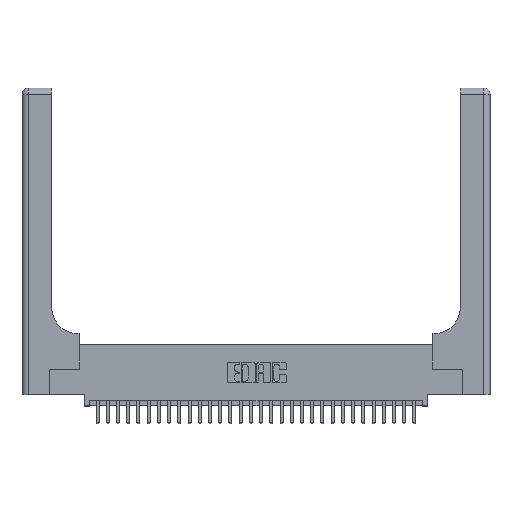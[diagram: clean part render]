
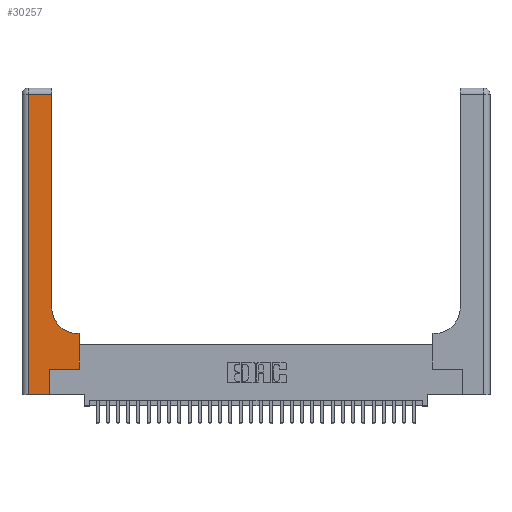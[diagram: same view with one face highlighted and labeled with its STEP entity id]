
A CAD part, top view. The second image highlights one B-rep face of the part: STEP entity #30257.
In plain terms, the highlighted planar face has unit normal (0, 0, 1).
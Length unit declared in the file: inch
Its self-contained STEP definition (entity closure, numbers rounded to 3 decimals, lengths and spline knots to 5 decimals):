
#98 = LINE ( 'NONE', #2803, #15893 ) ;
#493 = LINE ( 'NONE', #10135, #31707 ) ;
#1180 = LINE ( 'NONE', #30720, #22722 ) ;
#1497 = LINE ( 'NONE', #11393, #26143 ) ;
#1631 = VERTEX_POINT ( 'NONE', #13397 ) ;
#1966 = EDGE_CURVE ( 'NONE', #18219, #19879, #5481, .T. ) ;
#2193 = VECTOR ( 'NONE', #12172, 39.37008 ) ;
#2440 = DIRECTION ( 'NONE',  ( -1., 0., 0. ) ) ;
#2803 = CARTESIAN_POINT ( 'NONE',  ( 0., 2.94, 0.37 ) ) ;
#2908 = LINE ( 'NONE', #3976, #29521 ) ;
#3976 = CARTESIAN_POINT ( 'NONE',  ( 0.2915, 0.6, 0.37 ) ) ;
#4558 = ORIENTED_EDGE ( 'NONE', *, *, #24170, .T. ) ;
#4812 = CARTESIAN_POINT ( 'NONE',  ( 0.2915, 2.94, 0.37 ) ) ;
#5339 = EDGE_LOOP ( 'NONE', ( #22541, #31617, #4558, #27419, #28797, #8984, #29464, #28355, #5643 ) ) ;
#5365 = EDGE_CURVE ( 'NONE', #22304, #18219, #493, .T. ) ;
#5481 = LINE ( 'NONE', #19418, #30897 ) ;
#5643 = ORIENTED_EDGE ( 'NONE', *, *, #7189, .T. ) ;
#7189 = EDGE_CURVE ( 'NONE', #8084, #9835, #25106, .T. ) ;
#7614 = CARTESIAN_POINT ( 'NONE',  ( 0.269, 0., 0.37 ) ) ;
#8084 = VERTEX_POINT ( 'NONE', #26641 ) ;
#8344 = VECTOR ( 'NONE', #30410, 39.37008 ) ;
#8361 = DIRECTION ( 'NONE',  ( 1., 0., 0. ) ) ;
#8540 = EDGE_CURVE ( 'NONE', #25011, #22304, #1497, .T. ) ;
#8787 = CARTESIAN_POINT ( 'NONE',  ( 0.5585, 0.25, 0.37 ) ) ;
#8984 = ORIENTED_EDGE ( 'NONE', *, *, #5365, .T. ) ;
#9571 = EDGE_CURVE ( 'NONE', #18099, #25011, #14919, .T. ) ;
#9835 = VERTEX_POINT ( 'NONE', #11762 ) ;
#10135 = CARTESIAN_POINT ( 'NONE',  ( 0.269, 0.25, 0.37 ) ) ;
#10941 = CARTESIAN_POINT ( 'NONE',  ( 0.5415, 0.85, 0.37 ) ) ;
#11393 = CARTESIAN_POINT ( 'NONE',  ( 0.269, 0., 0.37 ) ) ;
#11762 = CARTESIAN_POINT ( 'NONE',  ( 0.2915, 0.85, 0.37 ) ) ;
#12172 = DIRECTION ( 'NONE',  ( 0., -1., 0. ) ) ;
#13397 = CARTESIAN_POINT ( 'NONE',  ( 0.06, 2.94, 0.37 ) ) ;
#14757 = DIRECTION ( 'NONE',  ( -1., 0., 0. ) ) ;
#14901 = DIRECTION ( 'NONE',  ( 0., 0., -1. ) ) ;
#14919 = LINE ( 'NONE', #22851, #8344 ) ;
#15893 = VECTOR ( 'NONE', #14757, 39.37008 ) ;
#17077 = CARTESIAN_POINT ( 'NONE',  ( 0., 3., 0.37 ) ) ;
#18026 = AXIS2_PLACEMENT_3D ( 'NONE', #17077, #14901, #2440 ) ;
#18099 = VERTEX_POINT ( 'NONE', #27879 ) ;
#18219 = VERTEX_POINT ( 'NONE', #8787 ) ;
#18425 = EDGE_CURVE ( 'NONE', #19879, #8084, #2908, .T. ) ;
#18727 = LINE ( 'NONE', #29206, #2193 ) ;
#19143 = DIRECTION ( 'NONE',  ( -1., 0., 0. ) ) ;
#19377 = CARTESIAN_POINT ( 'NONE',  ( 0.5585, 0.6, 0.37 ) ) ;
#19418 = CARTESIAN_POINT ( 'NONE',  ( 0.5585, 0.25, 0.37 ) ) ;
#19879 = VERTEX_POINT ( 'NONE', #19377 ) ;
#20010 = EDGE_CURVE ( 'NONE', #29647, #1631, #98, .T. ) ;
#20941 = EDGE_CURVE ( 'NONE', #9835, #29647, #1180, .T. ) ;
#22304 = VERTEX_POINT ( 'NONE', #28867 ) ;
#22328 = AXIS2_PLACEMENT_3D ( 'NONE', #10941, #23090, #8361 ) ;
#22541 = ORIENTED_EDGE ( 'NONE', *, *, #20941, .T. ) ;
#22722 = VECTOR ( 'NONE', #25664, 39.37008 ) ;
#22851 = CARTESIAN_POINT ( 'NONE',  ( 0., 0., 0.37 ) ) ;
#23090 = DIRECTION ( 'NONE',  ( 0., 0., -1. ) ) ;
#24001 = DIRECTION ( 'NONE',  ( 0., 1., 0. ) ) ;
#24170 = EDGE_CURVE ( 'NONE', #1631, #18099, #18727, .T. ) ;
#25011 = VERTEX_POINT ( 'NONE', #7614 ) ;
#25106 = CIRCLE ( 'NONE', #22328, 0.25 ) ;
#25664 = DIRECTION ( 'NONE',  ( 0., 1., 0. ) ) ;
#26143 = VECTOR ( 'NONE', #24001, 39.37008 ) ;
#26641 = CARTESIAN_POINT ( 'NONE',  ( 0.5415, 0.6, 0.37 ) ) ;
#27174 = DIRECTION ( 'NONE',  ( 1., 0., 0. ) ) ;
#27188 = PLANE ( 'NONE',  #18026 ) ;
#27419 = ORIENTED_EDGE ( 'NONE', *, *, #9571, .T. ) ;
#27879 = CARTESIAN_POINT ( 'NONE',  ( 0.06, 0., 0.37 ) ) ;
#28355 = ORIENTED_EDGE ( 'NONE', *, *, #18425, .T. ) ;
#28797 = ORIENTED_EDGE ( 'NONE', *, *, #8540, .T. ) ;
#28867 = CARTESIAN_POINT ( 'NONE',  ( 0.269, 0.25, 0.37 ) ) ;
#29114 = DIRECTION ( 'NONE',  ( 0., 1., 0. ) ) ;
#29206 = CARTESIAN_POINT ( 'NONE',  ( 0.06, 3., 0.37 ) ) ;
#29464 = ORIENTED_EDGE ( 'NONE', *, *, #1966, .T. ) ;
#29521 = VECTOR ( 'NONE', #19143, 39.37008 ) ;
#29647 = VERTEX_POINT ( 'NONE', #4812 ) ;
#30257 = ADVANCED_FACE ( 'NONE', ( #30677 ), #27188, .F. ) ;
#30410 = DIRECTION ( 'NONE',  ( 1., 0., 0. ) ) ;
#30677 = FACE_OUTER_BOUND ( 'NONE', #5339, .T. ) ;
#30720 = CARTESIAN_POINT ( 'NONE',  ( 0.2915, 3., 0.37 ) ) ;
#30897 = VECTOR ( 'NONE', #29114, 39.37008 ) ;
#31617 = ORIENTED_EDGE ( 'NONE', *, *, #20010, .T. ) ;
#31707 = VECTOR ( 'NONE', #27174, 39.37008 ) ;
